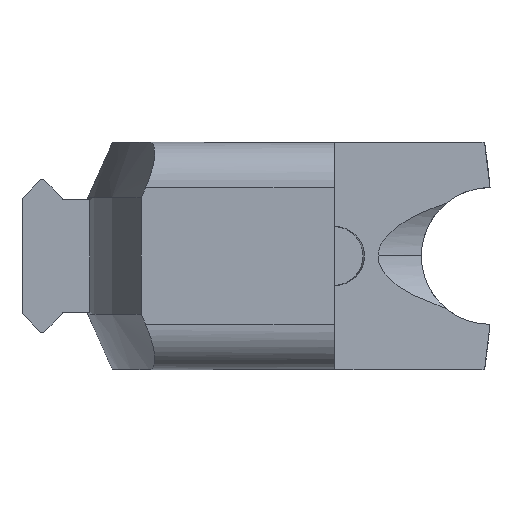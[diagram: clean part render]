
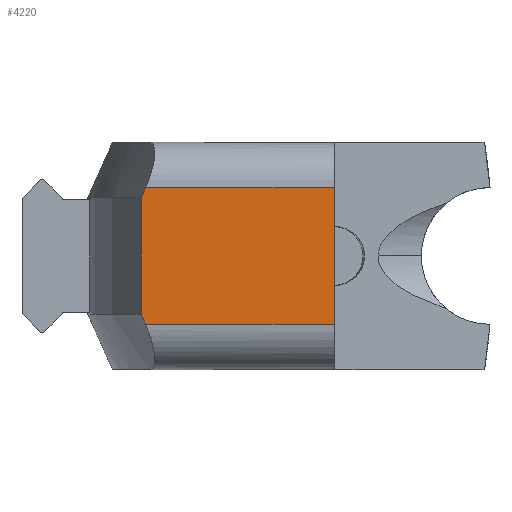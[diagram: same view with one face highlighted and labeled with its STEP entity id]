
A CAD part, left-side view. The second image highlights one B-rep face of the part: STEP entity #4220.
In plain terms, the highlighted planar face has unit normal (-1, 0, 0).
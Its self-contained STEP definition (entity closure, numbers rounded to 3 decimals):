
#141 = ORIENTED_EDGE ( 'NONE', *, *, #7650, .F. ) ;
#142 = DIRECTION ( 'NONE',  ( 0., -1., 0. ) ) ;
#483 = LINE ( 'NONE', #1804, #2200 ) ;
#579 = VERTEX_POINT ( 'NONE', #753 ) ;
#596 = EDGE_CURVE ( 'NONE', #579, #1367, #1061, .T. ) ;
#727 = AXIS2_PLACEMENT_3D ( 'NONE', #4558, #1983, #6488 ) ;
#753 = CARTESIAN_POINT ( 'NONE',  ( -3.834, 114.754, 168.134 ) ) ;
#891 = LINE ( 'NONE', #7666, #4533 ) ;
#1061 = LINE ( 'NONE', #7072, #2778 ) ;
#1336 = PLANE ( 'NONE',  #727 ) ;
#1367 = VERTEX_POINT ( 'NONE', #7500 ) ;
#1719 = CARTESIAN_POINT ( 'NONE',  ( -3.834, 141.69, 166.742 ) ) ;
#1738 = EDGE_LOOP ( 'NONE', ( #2444, #141, #4652, #6706, #2876, #4170 ) ) ;
#1804 = CARTESIAN_POINT ( 'NONE',  ( -3.834, 141.69, 150.476 ) ) ;
#1824 = VECTOR ( 'NONE', #142, 1000. ) ;
#1983 = DIRECTION ( 'NONE',  ( -1., 0., 0. ) ) ;
#2200 = VECTOR ( 'NONE', #6956, 1000. ) ;
#2341 = CARTESIAN_POINT ( 'NONE',  ( -3.834, 141.69, 158.609 ) ) ;
#2441 = LINE ( 'NONE', #2341, #2639 ) ;
#2444 = ORIENTED_EDGE ( 'NONE', *, *, #4323, .T. ) ;
#2639 = VECTOR ( 'NONE', #7482, 1000. ) ;
#2662 = VERTEX_POINT ( 'NONE', #5994 ) ;
#2778 = VECTOR ( 'NONE', #5786, 1000. ) ;
#2836 = FACE_OUTER_BOUND ( 'NONE', #1738, .T. ) ;
#2876 = ORIENTED_EDGE ( 'NONE', *, *, #3707, .T. ) ;
#2997 = VERTEX_POINT ( 'NONE', #6049 ) ;
#3109 = VECTOR ( 'NONE', #4495, 1000. ) ;
#3311 = LINE ( 'NONE', #7046, #3109 ) ;
#3707 = EDGE_CURVE ( 'NONE', #5378, #5602, #2441, .T. ) ;
#3739 = LINE ( 'NONE', #7873, #1824 ) ;
#3819 = DIRECTION ( 'NONE',  ( 0., -0.407, 0.914 ) ) ;
#4170 = ORIENTED_EDGE ( 'NONE', *, *, #8095, .T. ) ;
#4220 = ADVANCED_FACE ( 'NONE', ( #2836 ), #1336, .T. ) ;
#4323 = EDGE_CURVE ( 'NONE', #2662, #2997, #3739, .T. ) ;
#4495 = DIRECTION ( 'NONE',  ( 0., 0., -1. ) ) ;
#4533 = VECTOR ( 'NONE', #3819, 1000. ) ;
#4558 = CARTESIAN_POINT ( 'NONE',  ( -3.834, 114.754, 149.084 ) ) ;
#4652 = ORIENTED_EDGE ( 'NONE', *, *, #596, .T. ) ;
#4770 = EDGE_CURVE ( 'NONE', #5378, #1367, #891, .T. ) ;
#5378 = VERTEX_POINT ( 'NONE', #1719 ) ;
#5596 = CARTESIAN_POINT ( 'NONE',  ( -3.834, 141.69, 150.476 ) ) ;
#5602 = VERTEX_POINT ( 'NONE', #5596 ) ;
#5786 = DIRECTION ( 'NONE',  ( 0., 1., 0. ) ) ;
#5994 = CARTESIAN_POINT ( 'NONE',  ( -3.834, 141.071, 149.084 ) ) ;
#6049 = CARTESIAN_POINT ( 'NONE',  ( -3.834, 114.754, 149.084 ) ) ;
#6488 = DIRECTION ( 'NONE',  ( 0., 0., 1. ) ) ;
#6706 = ORIENTED_EDGE ( 'NONE', *, *, #4770, .F. ) ;
#6956 = DIRECTION ( 'NONE',  ( 0., -0.407, -0.914 ) ) ;
#7046 = CARTESIAN_POINT ( 'NONE',  ( -3.834, 114.754, 158.609 ) ) ;
#7072 = CARTESIAN_POINT ( 'NONE',  ( -3.834, 127.991, 168.134 ) ) ;
#7482 = DIRECTION ( 'NONE',  ( 0., 0., -1. ) ) ;
#7500 = CARTESIAN_POINT ( 'NONE',  ( -3.834, 141.071, 168.134 ) ) ;
#7650 = EDGE_CURVE ( 'NONE', #579, #2997, #3311, .T. ) ;
#7666 = CARTESIAN_POINT ( 'NONE',  ( -3.834, 139.971, 170.604 ) ) ;
#7873 = CARTESIAN_POINT ( 'NONE',  ( -3.834, 127.991, 149.084 ) ) ;
#8095 = EDGE_CURVE ( 'NONE', #5602, #2662, #483, .T. ) ;
